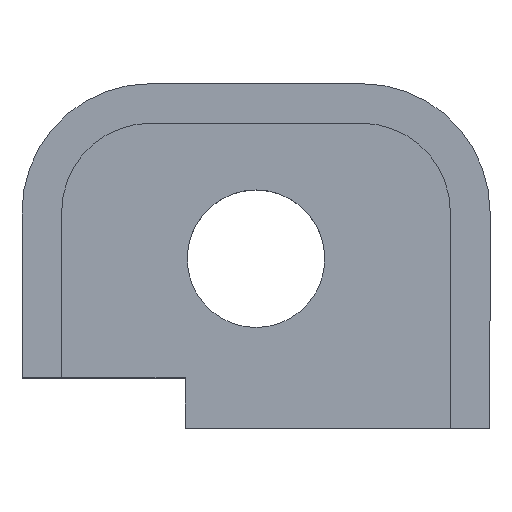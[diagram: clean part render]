
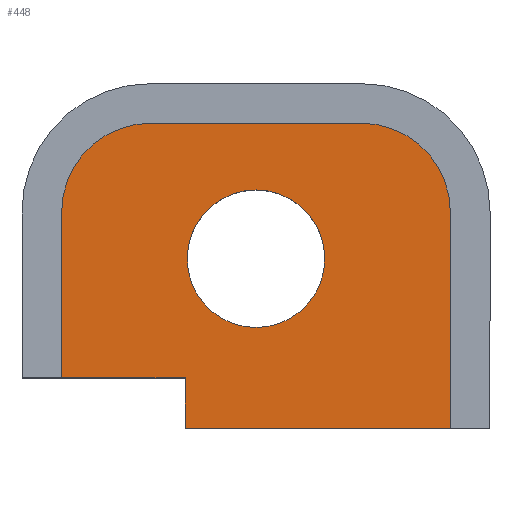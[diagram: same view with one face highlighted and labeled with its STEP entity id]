
A CAD part, top view. The second image highlights one B-rep face of the part: STEP entity #448.
In plain terms, the highlighted planar face has unit normal (0, 0, 1).
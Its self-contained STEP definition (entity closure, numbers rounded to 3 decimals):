
#29 = VECTOR ( 'NONE', #102, 1000. ) ;
#36 = EDGE_LOOP ( 'NONE', ( #51, #434, #507, #401, #160, #39, #381, #269 ) ) ;
#39 = ORIENTED_EDGE ( 'NONE', *, *, #192, .T. ) ;
#51 = ORIENTED_EDGE ( 'NONE', *, *, #187, .T. ) ;
#55 = CARTESIAN_POINT ( 'NONE',  ( -6.96, 7.747, 0. ) ) ;
#61 = EDGE_CURVE ( 'NONE', #278, #263, #346, .T. ) ;
#71 = CARTESIAN_POINT ( 'NONE',  ( -2.54, 1.803, 0. ) ) ;
#74 = VERTEX_POINT ( 'NONE', #470 ) ;
#88 = DIRECTION ( 'NONE',  ( 1., 0., 0. ) ) ;
#94 = ORIENTED_EDGE ( 'NONE', *, *, #597, .F. ) ;
#100 = CARTESIAN_POINT ( 'NONE',  ( -2.54, 0., 0. ) ) ;
#102 = DIRECTION ( 'NONE',  ( -1., 0., 0. ) ) ;
#110 = DIRECTION ( 'NONE',  ( 1., 0., 0. ) ) ;
#112 = CARTESIAN_POINT ( 'NONE',  ( -6.96, 7.747, 0. ) ) ;
#116 = CIRCLE ( 'NONE', #368, 3.175 ) ;
#117 = DIRECTION ( 'NONE',  ( 0., 0., 1. ) ) ;
#120 = AXIS2_PLACEMENT_3D ( 'NONE', #121, #117, #110 ) ;
#121 = CARTESIAN_POINT ( 'NONE',  ( 0., 6.071, 0. ) ) ;
#125 = LINE ( 'NONE', #350, #232 ) ;
#127 = EDGE_LOOP ( 'NONE', ( #291, #94 ) ) ;
#132 = EDGE_CURVE ( 'NONE', #208, #337, #526, .T. ) ;
#141 = AXIS2_PLACEMENT_3D ( 'NONE', #186, #183, #181 ) ;
#160 = ORIENTED_EDGE ( 'NONE', *, *, #132, .T. ) ;
#163 = EDGE_CURVE ( 'NONE', #263, #208, #116, .T. ) ;
#164 = EDGE_CURVE ( 'NONE', #437, #278, #228, .T. ) ;
#181 = DIRECTION ( 'NONE',  ( 1., 0., 0. ) ) ;
#183 = DIRECTION ( 'NONE',  ( 0., 0., 1. ) ) ;
#186 = CARTESIAN_POINT ( 'NONE',  ( 0., 6.071, 0. ) ) ;
#187 = EDGE_CURVE ( 'NONE', #421, #437, #125, .T. ) ;
#189 = VECTOR ( 'NONE', #575, 1000. ) ;
#192 = EDGE_CURVE ( 'NONE', #337, #610, #374, .T. ) ;
#205 = CARTESIAN_POINT ( 'NONE',  ( -2.54, 0., 0. ) ) ;
#208 = VERTEX_POINT ( 'NONE', #55 ) ;
#209 = VERTEX_POINT ( 'NONE', #205 ) ;
#223 = AXIS2_PLACEMENT_3D ( 'NONE', #377, #340, #320 ) ;
#228 = CIRCLE ( 'NONE', #400, 3.175 ) ;
#232 = VECTOR ( 'NONE', #322, 1000. ) ;
#246 = DIRECTION ( 'NONE',  ( 1., 0., 0. ) ) ;
#263 = VERTEX_POINT ( 'NONE', #567 ) ;
#269 = ORIENTED_EDGE ( 'NONE', *, *, #600, .T. ) ;
#278 = VERTEX_POINT ( 'NONE', #549 ) ;
#291 = ORIENTED_EDGE ( 'NONE', *, *, #561, .F. ) ;
#304 = CARTESIAN_POINT ( 'NONE',  ( -8.382, 1.803, 0. ) ) ;
#310 = EDGE_CURVE ( 'NONE', #610, #209, #568, .T. ) ;
#319 = CARTESIAN_POINT ( 'NONE',  ( -2.464, 6.071, 0. ) ) ;
#320 = DIRECTION ( 'NONE',  ( -1., 0., 0. ) ) ;
#322 = DIRECTION ( 'NONE',  ( 0., 1., 0. ) ) ;
#325 = VECTOR ( 'NONE', #246, 1000. ) ;
#328 = PLANE ( 'NONE',  #223 ) ;
#337 = VERTEX_POINT ( 'NONE', #465 ) ;
#340 = DIRECTION ( 'NONE',  ( 0., 0., -1. ) ) ;
#341 = CARTESIAN_POINT ( 'NONE',  ( 3.785, 7.747, 0. ) ) ;
#346 = LINE ( 'NONE', #415, #29 ) ;
#350 = CARTESIAN_POINT ( 'NONE',  ( 6.96, 0., 0. ) ) ;
#368 = AXIS2_PLACEMENT_3D ( 'NONE', #447, #425, #372 ) ;
#372 = DIRECTION ( 'NONE',  ( 1., 0., 0. ) ) ;
#374 = LINE ( 'NONE', #304, #325 ) ;
#376 = CARTESIAN_POINT ( 'NONE',  ( 6.96, 7.747, 0. ) ) ;
#377 = CARTESIAN_POINT ( 'NONE',  ( 3.785, 7.747, 0. ) ) ;
#381 = ORIENTED_EDGE ( 'NONE', *, *, #310, .T. ) ;
#393 = CARTESIAN_POINT ( 'NONE',  ( 6.96, 0., 0. ) ) ;
#400 = AXIS2_PLACEMENT_3D ( 'NONE', #341, #419, #422 ) ;
#401 = ORIENTED_EDGE ( 'NONE', *, *, #163, .T. ) ;
#415 = CARTESIAN_POINT ( 'NONE',  ( 3.785, 10.922, 0. ) ) ;
#419 = DIRECTION ( 'NONE',  ( 0., 0., 1. ) ) ;
#421 = VERTEX_POINT ( 'NONE', #393 ) ;
#422 = DIRECTION ( 'NONE',  ( 1., 0., 0. ) ) ;
#425 = DIRECTION ( 'NONE',  ( 0., 0., 1. ) ) ;
#434 = ORIENTED_EDGE ( 'NONE', *, *, #164, .T. ) ;
#437 = VERTEX_POINT ( 'NONE', #376 ) ;
#447 = CARTESIAN_POINT ( 'NONE',  ( -3.785, 7.747, 0. ) ) ;
#448 = ADVANCED_FACE ( 'NONE', ( #473, #586 ), #328, .F. ) ;
#465 = CARTESIAN_POINT ( 'NONE',  ( -6.96, 1.803, 0. ) ) ;
#470 = CARTESIAN_POINT ( 'NONE',  ( 2.464, 6.071, 0. ) ) ;
#473 = FACE_BOUND ( 'NONE', #127, .T. ) ;
#484 = DIRECTION ( 'NONE',  ( 0., -1., 0. ) ) ;
#495 = CIRCLE ( 'NONE', #120, 2.464 ) ;
#503 = CARTESIAN_POINT ( 'NONE',  ( -2.54, 1.803, 0. ) ) ;
#507 = ORIENTED_EDGE ( 'NONE', *, *, #61, .T. ) ;
#508 = VERTEX_POINT ( 'NONE', #319 ) ;
#526 = LINE ( 'NONE', #112, #189 ) ;
#547 = VECTOR ( 'NONE', #88, 1000. ) ;
#549 = CARTESIAN_POINT ( 'NONE',  ( 3.785, 10.922, 0. ) ) ;
#551 = CIRCLE ( 'NONE', #141, 2.464 ) ;
#561 = EDGE_CURVE ( 'NONE', #74, #508, #551, .T. ) ;
#563 = LINE ( 'NONE', #100, #547 ) ;
#567 = CARTESIAN_POINT ( 'NONE',  ( -3.785, 10.922, 0. ) ) ;
#568 = LINE ( 'NONE', #503, #603 ) ;
#575 = DIRECTION ( 'NONE',  ( 0., -1., 0. ) ) ;
#586 = FACE_OUTER_BOUND ( 'NONE', #36, .T. ) ;
#597 = EDGE_CURVE ( 'NONE', #508, #74, #495, .T. ) ;
#600 = EDGE_CURVE ( 'NONE', #209, #421, #563, .T. ) ;
#603 = VECTOR ( 'NONE', #484, 1000. ) ;
#610 = VERTEX_POINT ( 'NONE', #71 ) ;
